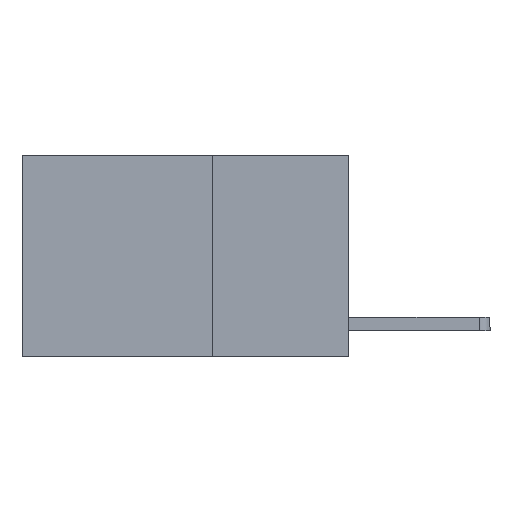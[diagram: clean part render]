
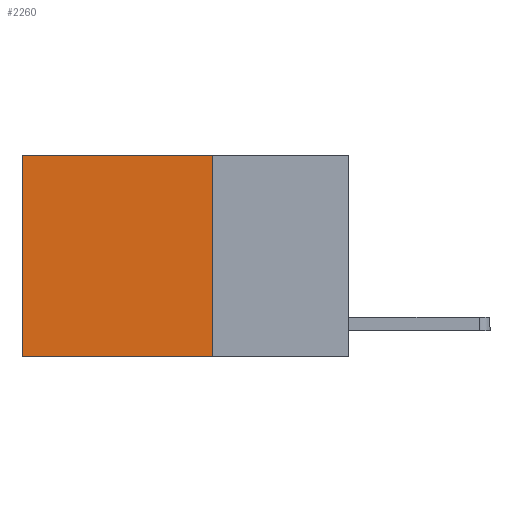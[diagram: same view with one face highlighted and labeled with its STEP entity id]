
A CAD part, left-side view. The second image highlights one B-rep face of the part: STEP entity #2260.
In plain terms, the highlighted planar face has unit normal (-1, 0, 0).
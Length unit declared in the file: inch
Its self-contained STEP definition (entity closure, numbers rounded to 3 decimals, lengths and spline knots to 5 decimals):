
#255 = CARTESIAN_POINT ( 'NONE',  ( 0.2625, 0.6, -0.37 ) ) ;
#475 = LINE ( 'NONE', #7804, #5951 ) ;
#739 = LINE ( 'NONE', #3352, #1540 ) ;
#1179 = ORIENTED_EDGE ( 'NONE', *, *, #3735, .T. ) ;
#1247 = LINE ( 'NONE', #3863, #8026 ) ;
#1540 = VECTOR ( 'NONE', #3946, 39.37008 ) ;
#1834 = CARTESIAN_POINT ( 'NONE',  ( 0.2625, 0.6, 0. ) ) ;
#2105 = ORIENTED_EDGE ( 'NONE', *, *, #3339, .F. ) ;
#2260 = ADVANCED_FACE ( 'NONE', ( #2346 ), #3432, .F. ) ;
#2346 = FACE_OUTER_BOUND ( 'NONE', #8367, .T. ) ;
#2518 = VECTOR ( 'NONE', #2537, 39.37008 ) ;
#2537 = DIRECTION ( 'NONE',  ( 0., 0., -1. ) ) ;
#2696 = CARTESIAN_POINT ( 'NONE',  ( 0.2625, 0.6, 0. ) ) ;
#2809 = CARTESIAN_POINT ( 'NONE',  ( 0.2625, 0.25, 0. ) ) ;
#3031 = DIRECTION ( 'NONE',  ( 1., 0., 0. ) ) ;
#3136 = ORIENTED_EDGE ( 'NONE', *, *, #3704, .T. ) ;
#3339 = EDGE_CURVE ( 'NONE', #5369, #5007, #1247, .T. ) ;
#3352 = CARTESIAN_POINT ( 'NONE',  ( 0.2625, 0.25, -0.37 ) ) ;
#3432 = PLANE ( 'NONE',  #6339 ) ;
#3456 = EDGE_CURVE ( 'NONE', #5007, #6167, #739, .T. ) ;
#3704 = EDGE_CURVE ( 'NONE', #7763, #6167, #8447, .T. ) ;
#3735 = EDGE_CURVE ( 'NONE', #5369, #7763, #475, .T. ) ;
#3863 = CARTESIAN_POINT ( 'NONE',  ( 0.2625, 0.25, 0. ) ) ;
#3946 = DIRECTION ( 'NONE',  ( 0., 1., 0. ) ) ;
#4802 = DIRECTION ( 'NONE',  ( 0., 0., -1. ) ) ;
#5007 = VERTEX_POINT ( 'NONE', #6017 ) ;
#5027 = DIRECTION ( 'NONE',  ( 0., 1., 0. ) ) ;
#5369 = VERTEX_POINT ( 'NONE', #2809 ) ;
#5951 = VECTOR ( 'NONE', #5027, 39.37008 ) ;
#6017 = CARTESIAN_POINT ( 'NONE',  ( 0.2625, 0.25, -0.37 ) ) ;
#6167 = VERTEX_POINT ( 'NONE', #255 ) ;
#6339 = AXIS2_PLACEMENT_3D ( 'NONE', #7410, #3031, #4802 ) ;
#6541 = ORIENTED_EDGE ( 'NONE', *, *, #3456, .F. ) ;
#6983 = DIRECTION ( 'NONE',  ( 0., 0., -1. ) ) ;
#7410 = CARTESIAN_POINT ( 'NONE',  ( 0.2625, 0.25, 0. ) ) ;
#7763 = VERTEX_POINT ( 'NONE', #2696 ) ;
#7804 = CARTESIAN_POINT ( 'NONE',  ( 0.2625, 0.25, 0. ) ) ;
#8026 = VECTOR ( 'NONE', #6983, 39.37008 ) ;
#8367 = EDGE_LOOP ( 'NONE', ( #3136, #6541, #2105, #1179 ) ) ;
#8447 = LINE ( 'NONE', #1834, #2518 ) ;
